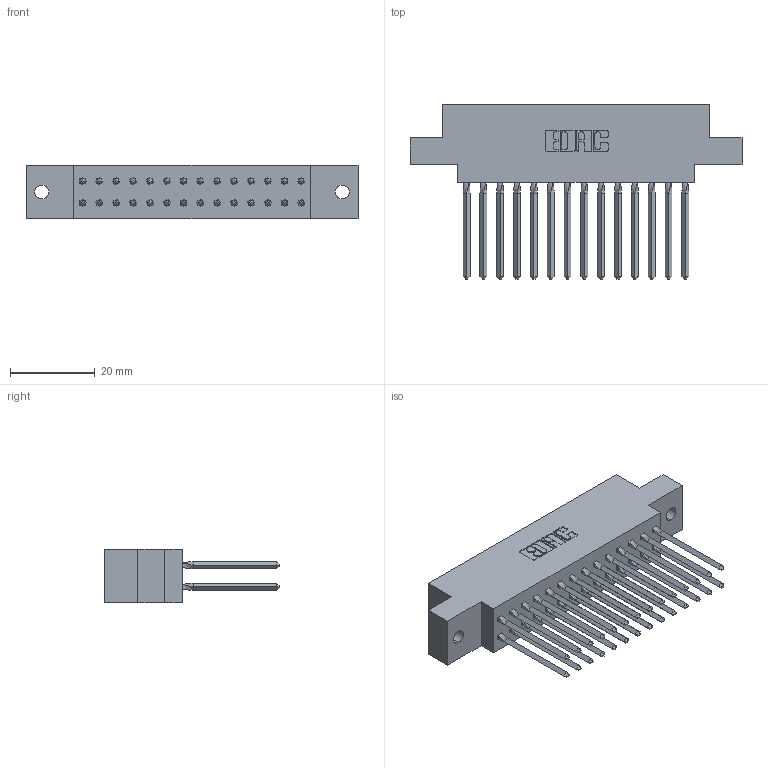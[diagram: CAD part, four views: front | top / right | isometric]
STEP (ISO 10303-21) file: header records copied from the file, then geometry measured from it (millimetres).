
FILE_DESCRIPTION (( 'STEP AP203' ), '1' );
FILE_NAME ('317-028-543-802.STEP', '2020-02-27T19:45:36', ( '' ), ( '' ), 'SwSTEP 2.0', 'SolidWorks 2016', '' );
FILE_SCHEMA (( 'CONFIG_CONTROL_DESIGN' ));
Length unit declared in the file: inch
Products named in the file (3): 317-028-543-802; 317-290-001_543; 317 Part_.144 Dia
Assembly tree (29 placements, depth 2):
  317-028-543-802
    317 Part_.144 Dia
    317-290-001_543  x28
Bounding box: 78.18 x 41.15 x 12.7 mm (x, y, z)
Volume: 12277.2 mm3; surface area: 17262.9 mm2
Topology: 29 solids, 29 shells, 2594 faces, 7191 edges, 4634 vertices
Faces by surface type: plane 2102, cylinder 380, bspline 112
Entity records: 24146 total; most frequent: CARTESIAN_POINT 4623, ORIENTED_EDGE 4122, DIRECTION 3443, EDGE_CURVE 2061, VECTOR 1805, LINE 1805, VERTEX_POINT 1367, AXIS2_PLACEMENT_3D 819
